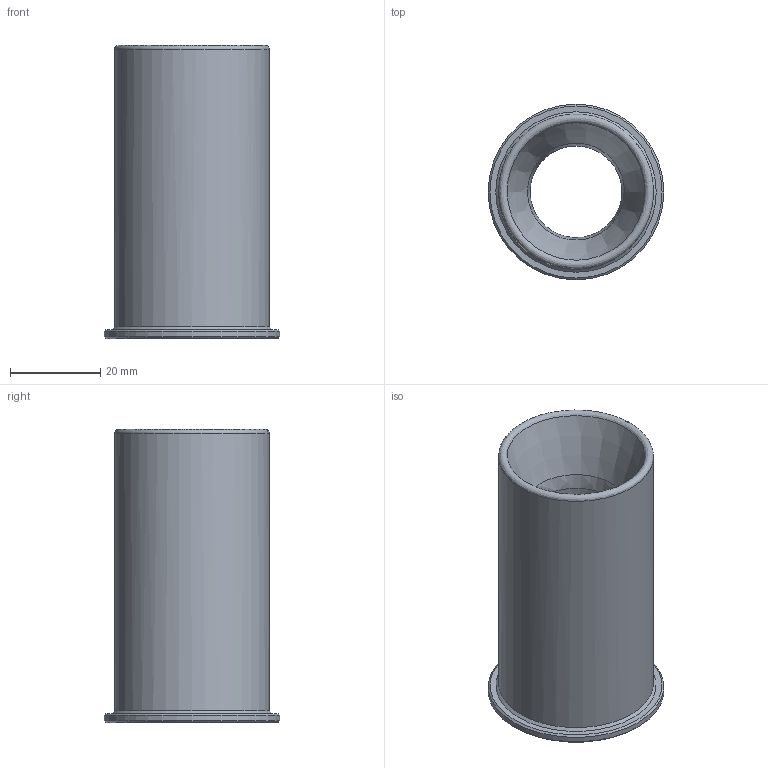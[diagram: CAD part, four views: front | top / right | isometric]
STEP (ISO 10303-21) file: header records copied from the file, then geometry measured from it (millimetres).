
FILE_DESCRIPTION(('FreeCAD Model'),'2;1');
FILE_NAME('Open CASCADE Shape Model','2022-10-05T16:46:44',('Author'),( ''),'Open CASCADE STEP processor 7.6','FreeCAD','Unknown');
FILE_SCHEMA(('AUTOMOTIVE_DESIGN { 1 0 10303 214 1 1 1 1 }'));
Length unit declared in the file: millimetre
Products named in the file (1): Case
Bounding box: 39 x 39 x 65.12 mm (x, y, z)
Volume: 36504.8 mm3; surface area: 12649.8 mm2
Topology: 1 solids, 1 shells, 16 faces, 29 edges, 16 vertices
Faces by surface type: cone 7, cylinder 4, plane 3, bspline 2
Full cylindrical faces by diameter (mm): 20.4 x1, 23 x1, 34.4 x1, 39 x1
Entity records: 1066 total; most frequent: CARTESIAN_POINT 468, DIRECTION 101, ORIENTED_EDGE 58, PCURVE 58, DEFINITIONAL_REPRESENTATION 58, LINE 43, VECTOR 43, EDGE_CURVE 29
